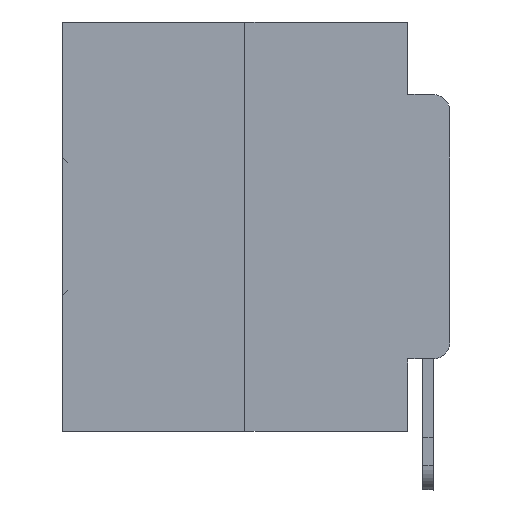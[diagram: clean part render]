
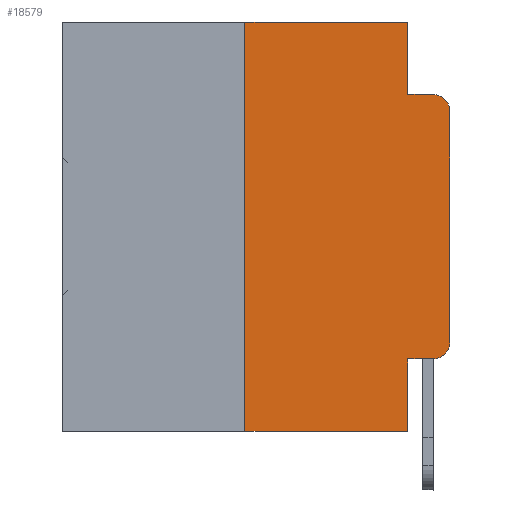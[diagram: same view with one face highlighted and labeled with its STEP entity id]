
A CAD part, left-side view. The second image highlights one B-rep face of the part: STEP entity #18579.
In plain terms, the highlighted planar face has unit normal (-1, 0, 0).
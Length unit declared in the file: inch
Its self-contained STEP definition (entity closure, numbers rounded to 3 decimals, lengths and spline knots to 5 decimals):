
#382 = EDGE_CURVE ( 'NONE', #29842, #9748, #29170, .T. ) ;
#778 = CARTESIAN_POINT ( 'NONE',  ( 0., 0.25, 0. ) ) ;
#1298 = CARTESIAN_POINT ( 'NONE',  ( 0., 0.051, 0. ) ) ;
#2052 = DIRECTION ( 'NONE',  ( 0., -1., 0. ) ) ;
#2867 = VECTOR ( 'NONE', #27648, 39.37008 ) ;
#2931 = VECTOR ( 'NONE', #7957, 39.37008 ) ;
#3110 = VECTOR ( 'NONE', #11134, 39.37008 ) ;
#3124 = ORIENTED_EDGE ( 'NONE', *, *, #7204, .F. ) ;
#3318 = DIRECTION ( 'NONE',  ( -1., 0., 0. ) ) ;
#4066 = LINE ( 'NONE', #1298, #2867 ) ;
#4243 = DIRECTION ( 'NONE',  ( 1., 0., 0. ) ) ;
#5183 = DIRECTION ( 'NONE',  ( -1., 0., 0. ) ) ;
#5708 = VERTEX_POINT ( 'NONE', #13489 ) ;
#5904 = EDGE_CURVE ( 'NONE', #9018, #9216, #29665, .T. ) ;
#6075 = CARTESIAN_POINT ( 'NONE',  ( 0., 0.051, 0. ) ) ;
#6570 = LINE ( 'NONE', #8485, #12084 ) ;
#6656 = DIRECTION ( 'NONE',  ( 0., 0., -1. ) ) ;
#7204 = EDGE_CURVE ( 'NONE', #12895, #23412, #18865, .T. ) ;
#7414 = CARTESIAN_POINT ( 'NONE',  ( 0., 0., -0.1085 ) ) ;
#7501 = LINE ( 'NONE', #17834, #12380 ) ;
#7745 = EDGE_CURVE ( 'NONE', #9216, #5708, #19982, .T. ) ;
#7828 = DIRECTION ( 'NONE',  ( 0., 0., 1. ) ) ;
#7957 = DIRECTION ( 'NONE',  ( 0., -1., 0. ) ) ;
#8485 = CARTESIAN_POINT ( 'NONE',  ( 0., 0.473, 0. ) ) ;
#8648 = CIRCLE ( 'NONE', #21837, 0.02 ) ;
#9018 = VERTEX_POINT ( 'NONE', #10095 ) ;
#9109 = VECTOR ( 'NONE', #11426, 39.37008 ) ;
#9202 = ORIENTED_EDGE ( 'NONE', *, *, #382, .T. ) ;
#9216 = VERTEX_POINT ( 'NONE', #30026 ) ;
#9662 = EDGE_CURVE ( 'NONE', #23412, #9018, #6570, .T. ) ;
#9748 = VERTEX_POINT ( 'NONE', #7414 ) ;
#10095 = CARTESIAN_POINT ( 'NONE',  ( 0., 0.051, 0. ) ) ;
#10371 = ORIENTED_EDGE ( 'NONE', *, *, #7745, .F. ) ;
#11134 = DIRECTION ( 'NONE',  ( 0., 0., 1. ) ) ;
#11426 = DIRECTION ( 'NONE',  ( 0., 0., -1. ) ) ;
#12084 = VECTOR ( 'NONE', #18971, 39.37008 ) ;
#12380 = VECTOR ( 'NONE', #25915, 39.37008 ) ;
#12588 = ORIENTED_EDGE ( 'NONE', *, *, #16559, .T. ) ;
#12895 = VERTEX_POINT ( 'NONE', #30421 ) ;
#12942 = CARTESIAN_POINT ( 'NONE',  ( 0., 0.02, -0.3915 ) ) ;
#13489 = CARTESIAN_POINT ( 'NONE',  ( 0., 0.02, -0.0885 ) ) ;
#14619 = VERTEX_POINT ( 'NONE', #25211 ) ;
#15826 = ORIENTED_EDGE ( 'NONE', *, *, #9662, .F. ) ;
#15875 = LINE ( 'NONE', #24136, #2931 ) ;
#15921 = CARTESIAN_POINT ( 'NONE',  ( 0., 0., 0. ) ) ;
#16559 = EDGE_CURVE ( 'NONE', #14619, #29842, #32470, .T. ) ;
#17026 = VECTOR ( 'NONE', #7828, 39.37008 ) ;
#17321 = FACE_OUTER_BOUND ( 'NONE', #27089, .T. ) ;
#17834 = CARTESIAN_POINT ( 'NONE',  ( 0., 0.473, -0.5 ) ) ;
#18530 = EDGE_CURVE ( 'NONE', #31501, #18551, #4066, .T. ) ;
#18546 = VECTOR ( 'NONE', #2052, 39.37008 ) ;
#18551 = VERTEX_POINT ( 'NONE', #27484 ) ;
#18579 = ADVANCED_FACE ( 'NONE', ( #17321 ), #19750, .F. ) ;
#18865 = LINE ( 'NONE', #778, #3110 ) ;
#18971 = DIRECTION ( 'NONE',  ( 0., -1., 0. ) ) ;
#19640 = CARTESIAN_POINT ( 'NONE',  ( 0., 0.051, -0.0885 ) ) ;
#19750 = PLANE ( 'NONE',  #26522 ) ;
#19982 = LINE ( 'NONE', #19640, #18546 ) ;
#20100 = ORIENTED_EDGE ( 'NONE', *, *, #28792, .T. ) ;
#20677 = ORIENTED_EDGE ( 'NONE', *, *, #5904, .F. ) ;
#21165 = CARTESIAN_POINT ( 'NONE',  ( 0., 0., -0.3915 ) ) ;
#21837 = AXIS2_PLACEMENT_3D ( 'NONE', #31896, #3318, #29149 ) ;
#22237 = ORIENTED_EDGE ( 'NONE', *, *, #24302, .T. ) ;
#22538 = EDGE_CURVE ( 'NONE', #12895, #18551, #7501, .T. ) ;
#23412 = VERTEX_POINT ( 'NONE', #31136 ) ;
#24049 = CARTESIAN_POINT ( 'NONE',  ( 0., 0.051, -0.4115 ) ) ;
#24136 = CARTESIAN_POINT ( 'NONE',  ( 0., 0.051, -0.4115 ) ) ;
#24246 = ORIENTED_EDGE ( 'NONE', *, *, #22538, .T. ) ;
#24302 = EDGE_CURVE ( 'NONE', #9748, #5708, #8648, .T. ) ;
#25211 = CARTESIAN_POINT ( 'NONE',  ( 0., 0.02, -0.4115 ) ) ;
#25915 = DIRECTION ( 'NONE',  ( 0., -1., 0. ) ) ;
#26522 = AXIS2_PLACEMENT_3D ( 'NONE', #30248, #4243, #6656 ) ;
#26531 = DIRECTION ( 'NONE',  ( 0., 0., -1. ) ) ;
#27089 = EDGE_LOOP ( 'NONE', ( #9202, #22237, #10371, #20677, #15826, #3124, #24246, #32911, #20100, #12588 ) ) ;
#27484 = CARTESIAN_POINT ( 'NONE',  ( 0., 0.051, -0.5 ) ) ;
#27648 = DIRECTION ( 'NONE',  ( 0., 0., -1. ) ) ;
#28792 = EDGE_CURVE ( 'NONE', #31501, #14619, #15875, .T. ) ;
#29149 = DIRECTION ( 'NONE',  ( 0., 0., -1. ) ) ;
#29170 = LINE ( 'NONE', #15921, #17026 ) ;
#29665 = LINE ( 'NONE', #6075, #9109 ) ;
#29729 = AXIS2_PLACEMENT_3D ( 'NONE', #12942, #5183, #26531 ) ;
#29842 = VERTEX_POINT ( 'NONE', #21165 ) ;
#30026 = CARTESIAN_POINT ( 'NONE',  ( 0., 0.051, -0.0885 ) ) ;
#30248 = CARTESIAN_POINT ( 'NONE',  ( 0., 0.473, 0. ) ) ;
#30421 = CARTESIAN_POINT ( 'NONE',  ( 0., 0.25, -0.5 ) ) ;
#31136 = CARTESIAN_POINT ( 'NONE',  ( 0., 0.25, 0. ) ) ;
#31501 = VERTEX_POINT ( 'NONE', #24049 ) ;
#31896 = CARTESIAN_POINT ( 'NONE',  ( 0., 0.02, -0.1085 ) ) ;
#32470 = CIRCLE ( 'NONE', #29729, 0.02 ) ;
#32911 = ORIENTED_EDGE ( 'NONE', *, *, #18530, .F. ) ;
